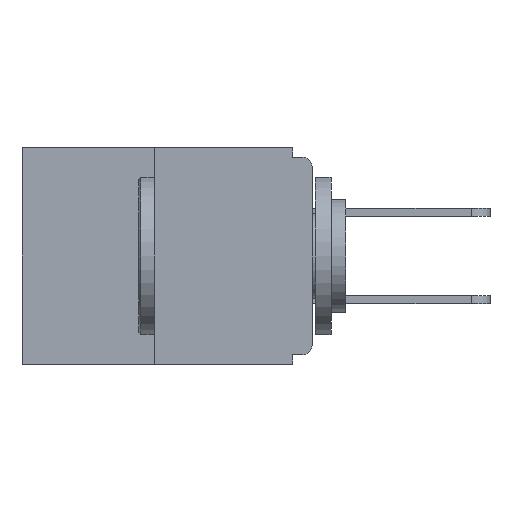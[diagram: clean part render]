
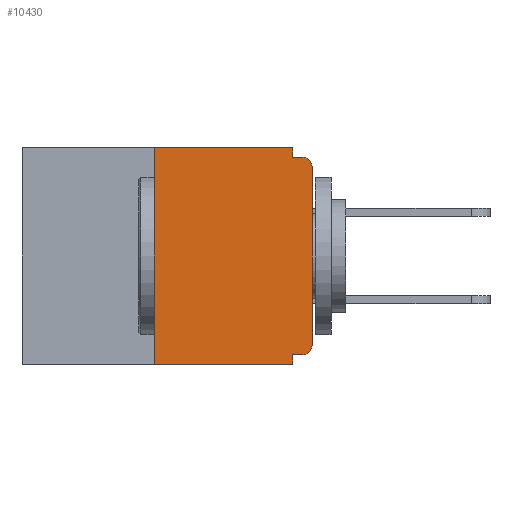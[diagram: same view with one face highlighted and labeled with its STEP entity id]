
A CAD part, left-side view. The second image highlights one B-rep face of the part: STEP entity #10430.
In plain terms, the highlighted planar face has unit normal (-1, 0, 0).
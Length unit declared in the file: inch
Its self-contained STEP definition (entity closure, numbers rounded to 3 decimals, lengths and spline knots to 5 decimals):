
#103 = CARTESIAN_POINT ( 'NONE',  ( 0., 0.25, 0. ) ) ;
#413 = ORIENTED_EDGE ( 'NONE', *, *, #20022, .F. ) ;
#450 = PLANE ( 'NONE',  #2853 ) ;
#755 = CARTESIAN_POINT ( 'NONE',  ( 0., 0., -0.015 ) ) ;
#1721 = EDGE_CURVE ( 'NONE', #21349, #16000, #5838, .T. ) ;
#1794 = ORIENTED_EDGE ( 'NONE', *, *, #5955, .F. ) ;
#1900 = EDGE_CURVE ( 'NONE', #19732, #10516, #4683, .T. ) ;
#2853 = AXIS2_PLACEMENT_3D ( 'NONE', #4056, #20575, #11290 ) ;
#3524 = CARTESIAN_POINT ( 'NONE',  ( 0., 0.031, -0.328 ) ) ;
#3525 = VECTOR ( 'NONE', #21035, 39.37008 ) ;
#3760 = CARTESIAN_POINT ( 'NONE',  ( 0., 0.031, 0. ) ) ;
#3854 = EDGE_CURVE ( 'NONE', #22728, #13503, #17976, .T. ) ;
#4056 = CARTESIAN_POINT ( 'NONE',  ( 0., 0.46, 0. ) ) ;
#4673 = ORIENTED_EDGE ( 'NONE', *, *, #10568, .F. ) ;
#4683 = CIRCLE ( 'NONE', #22859, 0.015 ) ;
#4709 = CARTESIAN_POINT ( 'NONE',  ( 0., 0., 0. ) ) ;
#4779 = EDGE_CURVE ( 'NONE', #9085, #21798, #23106, .T. ) ;
#4998 = CARTESIAN_POINT ( 'NONE',  ( 0., 0.46, -0.343 ) ) ;
#5536 = CARTESIAN_POINT ( 'NONE',  ( 0., 0.031, -0.343 ) ) ;
#5838 = LINE ( 'NONE', #5536, #8948 ) ;
#5955 = EDGE_CURVE ( 'NONE', #13503, #19755, #7641, .T. ) ;
#6363 = DIRECTION ( 'NONE',  ( 0., 0., -1. ) ) ;
#6523 = DIRECTION ( 'NONE',  ( 0., 0., 1. ) ) ;
#6762 = CARTESIAN_POINT ( 'NONE',  ( 0., 0.25, 0. ) ) ;
#7026 = ORIENTED_EDGE ( 'NONE', *, *, #3854, .F. ) ;
#7379 = ORIENTED_EDGE ( 'NONE', *, *, #1721, .F. ) ;
#7454 = VECTOR ( 'NONE', #10379, 39.37008 ) ;
#7641 = LINE ( 'NONE', #11481, #9976 ) ;
#7773 = VERTEX_POINT ( 'NONE', #10387 ) ;
#7954 = LINE ( 'NONE', #4709, #11108 ) ;
#8948 = VECTOR ( 'NONE', #21933, 39.37008 ) ;
#9031 = CARTESIAN_POINT ( 'NONE',  ( 0., 0.015, -0.313 ) ) ;
#9085 = VERTEX_POINT ( 'NONE', #22568 ) ;
#9976 = VECTOR ( 'NONE', #18700, 39.37008 ) ;
#10027 = DIRECTION ( 'NONE',  ( 0., -1., 0. ) ) ;
#10265 = ORIENTED_EDGE ( 'NONE', *, *, #1900, .T. ) ;
#10305 = LINE ( 'NONE', #4998, #14570 ) ;
#10349 = LINE ( 'NONE', #755, #19723 ) ;
#10379 = DIRECTION ( 'NONE',  ( 0., 0., 1. ) ) ;
#10387 = CARTESIAN_POINT ( 'NONE',  ( 0., 0.25, -0.343 ) ) ;
#10430 = ADVANCED_FACE ( 'NONE', ( #15231 ), #450, .F. ) ;
#10516 = VERTEX_POINT ( 'NONE', #13748 ) ;
#10568 = EDGE_CURVE ( 'NONE', #19755, #10516, #10349, .T. ) ;
#11108 = VECTOR ( 'NONE', #6523, 39.37008 ) ;
#11121 = AXIS2_PLACEMENT_3D ( 'NONE', #9031, #21690, #12802 ) ;
#11290 = DIRECTION ( 'NONE',  ( 0., 0., -1. ) ) ;
#11405 = ORIENTED_EDGE ( 'NONE', *, *, #22889, .T. ) ;
#11481 = CARTESIAN_POINT ( 'NONE',  ( 0., 0.031, 0. ) ) ;
#11782 = LINE ( 'NONE', #6762, #7454 ) ;
#11842 = CARTESIAN_POINT ( 'NONE',  ( 0., 0., -0.328 ) ) ;
#12277 = EDGE_LOOP ( 'NONE', ( #7026, #14771, #11405, #7379, #413, #19776, #17797, #10265, #4673, #1794 ) ) ;
#12802 = DIRECTION ( 'NONE',  ( 0., 0., -1. ) ) ;
#12841 = EDGE_CURVE ( 'NONE', #21798, #19732, #7954, .T. ) ;
#13386 = CARTESIAN_POINT ( 'NONE',  ( 0., 0.46, 0. ) ) ;
#13503 = VERTEX_POINT ( 'NONE', #3760 ) ;
#13748 = CARTESIAN_POINT ( 'NONE',  ( 0., 0.015, -0.015 ) ) ;
#13765 = LINE ( 'NONE', #11842, #3525 ) ;
#14122 = CARTESIAN_POINT ( 'NONE',  ( 0., 0., -0.03 ) ) ;
#14570 = VECTOR ( 'NONE', #17725, 39.37008 ) ;
#14768 = CARTESIAN_POINT ( 'NONE',  ( 0., 0.031, -0.015 ) ) ;
#14771 = ORIENTED_EDGE ( 'NONE', *, *, #20156, .F. ) ;
#15231 = FACE_OUTER_BOUND ( 'NONE', #12277, .T. ) ;
#16000 = VERTEX_POINT ( 'NONE', #22957 ) ;
#16735 = CARTESIAN_POINT ( 'NONE',  ( 0., 0., -0.313 ) ) ;
#17430 = DIRECTION ( 'NONE',  ( -1., 0., 0. ) ) ;
#17725 = DIRECTION ( 'NONE',  ( 0., -1., 0. ) ) ;
#17797 = ORIENTED_EDGE ( 'NONE', *, *, #12841, .T. ) ;
#17976 = LINE ( 'NONE', #13386, #22436 ) ;
#18700 = DIRECTION ( 'NONE',  ( 0., 0., -1. ) ) ;
#19723 = VECTOR ( 'NONE', #10027, 39.37008 ) ;
#19732 = VERTEX_POINT ( 'NONE', #14122 ) ;
#19755 = VERTEX_POINT ( 'NONE', #14768 ) ;
#19776 = ORIENTED_EDGE ( 'NONE', *, *, #4779, .T. ) ;
#20022 = EDGE_CURVE ( 'NONE', #9085, #21349, #13765, .T. ) ;
#20156 = EDGE_CURVE ( 'NONE', #7773, #22728, #11782, .T. ) ;
#20291 = DIRECTION ( 'NONE',  ( 0., -1., 0. ) ) ;
#20575 = DIRECTION ( 'NONE',  ( 1., 0., 0. ) ) ;
#21035 = DIRECTION ( 'NONE',  ( 0., 1., 0. ) ) ;
#21349 = VERTEX_POINT ( 'NONE', #3524 ) ;
#21690 = DIRECTION ( 'NONE',  ( -1., 0., 0. ) ) ;
#21798 = VERTEX_POINT ( 'NONE', #16735 ) ;
#21933 = DIRECTION ( 'NONE',  ( 0., 0., -1. ) ) ;
#22436 = VECTOR ( 'NONE', #20291, 39.37008 ) ;
#22520 = CARTESIAN_POINT ( 'NONE',  ( 0., 0.015, -0.03 ) ) ;
#22568 = CARTESIAN_POINT ( 'NONE',  ( 0., 0.015, -0.328 ) ) ;
#22728 = VERTEX_POINT ( 'NONE', #103 ) ;
#22859 = AXIS2_PLACEMENT_3D ( 'NONE', #22520, #17430, #6363 ) ;
#22889 = EDGE_CURVE ( 'NONE', #7773, #16000, #10305, .T. ) ;
#22957 = CARTESIAN_POINT ( 'NONE',  ( 0., 0.031, -0.343 ) ) ;
#23106 = CIRCLE ( 'NONE', #11121, 0.015 ) ;
